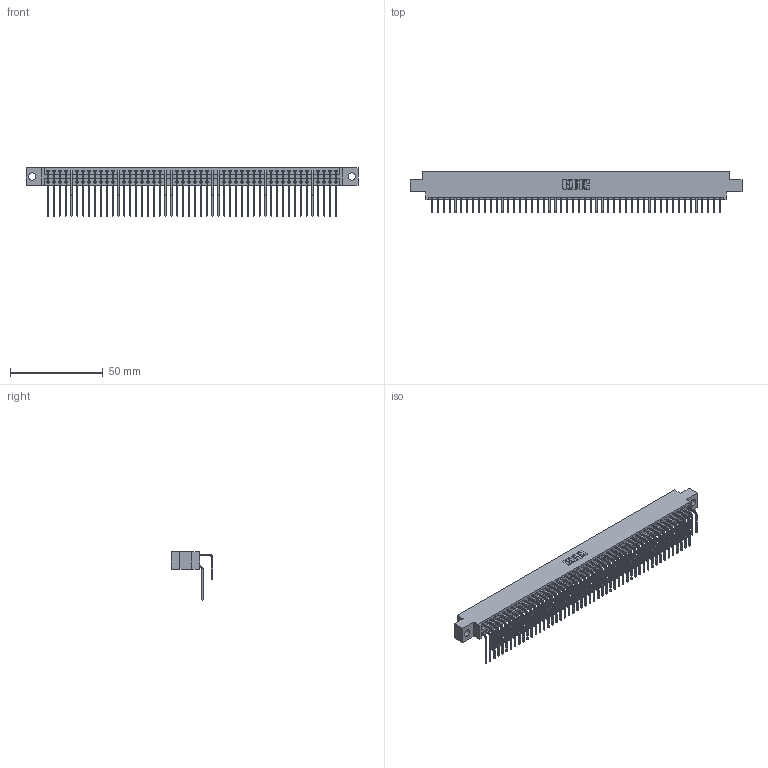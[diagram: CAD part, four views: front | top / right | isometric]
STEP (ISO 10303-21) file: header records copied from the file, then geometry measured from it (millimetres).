
FILE_DESCRIPTION (( 'STEP AP203' ), '1' );
FILE_NAME ('346-100-558-804.STEP', '2022-05-26T21:26:20', ( '' ), ( '' ), 'SwSTEP 2.0', 'SolidWorks 2020', '' );
FILE_SCHEMA (( 'CONFIG_CONTROL_DESIGN' ));
Length unit declared in the file: inch
Products named in the file (4): 345-292-001_558 559 Tail - 1; 346 Part_0.170 Offset - 0.156 Dia-TH; 346-100-558-804; 345-292-001_558 Tail - 2
Assembly tree (101 placements, depth 2):
  346-100-558-804
    346 Part_0.170 Offset - 0.156 Dia-TH
    345-292-001_558 559 Tail - 1  x50
    345-292-001_558 Tail - 2  x50
Bounding box: 179.32 x 22.16 x 26.16 mm (x, y, z)
Volume: 17864.8 mm3; surface area: 27477 mm2
Topology: 101 solids, 101 shells, 5540 faces, 16477 edges, 10850 vertices
Faces by surface type: plane 3794, cylinder 1746
Entity records: 33889 total; most frequent: CARTESIAN_POINT 5633, ORIENTED_EDGE 5514, DIRECTION 4985, EDGE_CURVE 2757, LINE 2385, VECTOR 2385, VERTEX_POINT 1834, AXIS2_PLACEMENT_3D 1300
